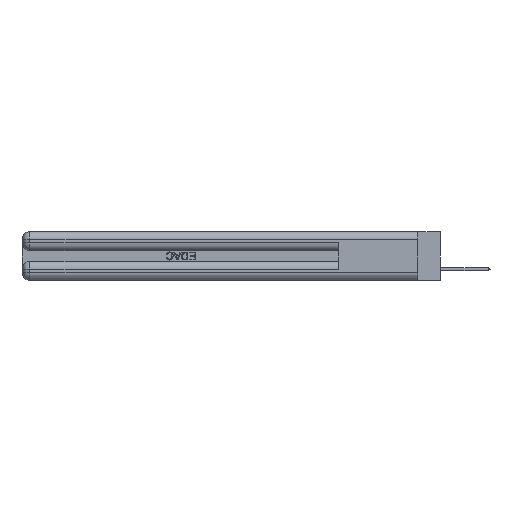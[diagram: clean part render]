
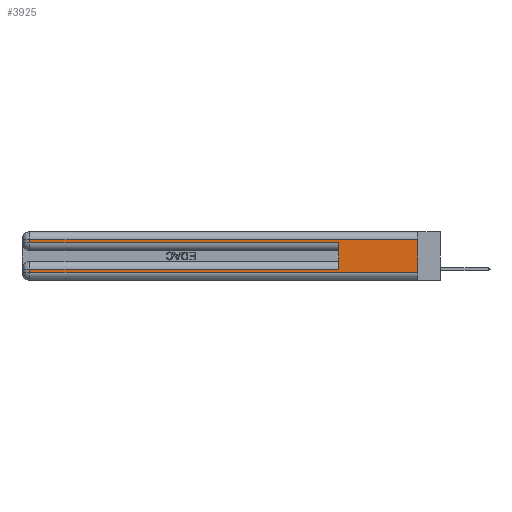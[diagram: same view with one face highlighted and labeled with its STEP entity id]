
A CAD part, left-side view. The second image highlights one B-rep face of the part: STEP entity #3925.
In plain terms, the highlighted planar face has unit normal (-1, 0, 0).
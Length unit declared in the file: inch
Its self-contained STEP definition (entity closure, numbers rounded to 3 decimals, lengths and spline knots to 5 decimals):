
#983 = ORIENTED_EDGE ( 'NONE', *, *, #35590, .T. ) ;
#3925 = ADVANCED_FACE ( 'NONE', ( #25614 ), #25757, .F. ) ;
#3992 = VERTEX_POINT ( 'NONE', #15371 ) ;
#4685 = DIRECTION ( 'NONE',  ( 0., 1., 0. ) ) ;
#4879 = CARTESIAN_POINT ( 'NONE',  ( 0., 2.94, 0.285 ) ) ;
#5951 = VERTEX_POINT ( 'NONE', #17149 ) ;
#6037 = VERTEX_POINT ( 'NONE', #38545 ) ;
#6633 = EDGE_CURVE ( 'NONE', #3992, #28101, #35765, .T. ) ;
#7548 = VERTEX_POINT ( 'NONE', #35885 ) ;
#9211 = LINE ( 'NONE', #29514, #38019 ) ;
#9677 = ORIENTED_EDGE ( 'NONE', *, *, #19985, .F. ) ;
#11271 = CARTESIAN_POINT ( 'NONE',  ( 0., 0., 0.37 ) ) ;
#12176 = EDGE_CURVE ( 'NONE', #13799, #7548, #9211, .T. ) ;
#12217 = DIRECTION ( 'NONE',  ( 0., 0., -1. ) ) ;
#12377 = DIRECTION ( 'NONE',  ( 0., 0., -1. ) ) ;
#12489 = LINE ( 'NONE', #27497, #17004 ) ;
#12563 = EDGE_CURVE ( 'NONE', #41067, #20176, #24419, .T. ) ;
#12713 = ORIENTED_EDGE ( 'NONE', *, *, #6633, .T. ) ;
#13020 = VECTOR ( 'NONE', #12377, 39.37008 ) ;
#13691 = CARTESIAN_POINT ( 'NONE',  ( 0., 0., 0.06 ) ) ;
#13745 = CARTESIAN_POINT ( 'NONE',  ( 0., 0.6, 0.285 ) ) ;
#13799 = VERTEX_POINT ( 'NONE', #23490 ) ;
#13914 = VECTOR ( 'NONE', #40086, 39.37008 ) ;
#14668 = EDGE_CURVE ( 'NONE', #7548, #3992, #42395, .T. ) ;
#14805 = VECTOR ( 'NONE', #18972, 39.37008 ) ;
#14844 = CARTESIAN_POINT ( 'NONE',  ( 0., 0.6, 0.145 ) ) ;
#15371 = CARTESIAN_POINT ( 'NONE',  ( 0., 2.94, 0.06 ) ) ;
#16921 = LINE ( 'NONE', #17027, #31066 ) ;
#17004 = VECTOR ( 'NONE', #45687, 39.37008 ) ;
#17027 = CARTESIAN_POINT ( 'NONE',  ( 0., 0., 0.31 ) ) ;
#17149 = CARTESIAN_POINT ( 'NONE',  ( 0., 0., 0.31 ) ) ;
#18445 = ORIENTED_EDGE ( 'NONE', *, *, #12176, .T. ) ;
#18704 = VECTOR ( 'NONE', #42557, 39.37008 ) ;
#18972 = DIRECTION ( 'NONE',  ( 0., -1., 0. ) ) ;
#19136 = CARTESIAN_POINT ( 'NONE',  ( 0., 0., 0.285 ) ) ;
#19985 = EDGE_CURVE ( 'NONE', #5951, #28101, #12489, .T. ) ;
#20176 = VERTEX_POINT ( 'NONE', #13745 ) ;
#22320 = LINE ( 'NONE', #14844, #13914 ) ;
#23490 = CARTESIAN_POINT ( 'NONE',  ( 0., 0.6, 0.085 ) ) ;
#23525 = EDGE_CURVE ( 'NONE', #13799, #20176, #22320, .T. ) ;
#24419 = LINE ( 'NONE', #19136, #14805 ) ;
#25614 = FACE_OUTER_BOUND ( 'NONE', #29400, .T. ) ;
#25757 = PLANE ( 'NONE',  #39024 ) ;
#25872 = ORIENTED_EDGE ( 'NONE', *, *, #12563, .T. ) ;
#26245 = LINE ( 'NONE', #45689, #26849 ) ;
#26849 = VECTOR ( 'NONE', #27986, 39.37008 ) ;
#27497 = CARTESIAN_POINT ( 'NONE',  ( 0., 0., 0.37 ) ) ;
#27986 = DIRECTION ( 'NONE',  ( 0., 0., -1. ) ) ;
#28101 = VERTEX_POINT ( 'NONE', #30935 ) ;
#29400 = EDGE_LOOP ( 'NONE', ( #9677, #983, #44951, #25872, #35628, #18445, #33652, #12713 ) ) ;
#29514 = CARTESIAN_POINT ( 'NONE',  ( 0., 0., 0.085 ) ) ;
#30935 = CARTESIAN_POINT ( 'NONE',  ( 0., 0., 0.06 ) ) ;
#31066 = VECTOR ( 'NONE', #42462, 39.37008 ) ;
#32209 = EDGE_CURVE ( 'NONE', #6037, #41067, #26245, .T. ) ;
#33652 = ORIENTED_EDGE ( 'NONE', *, *, #14668, .T. ) ;
#33838 = DIRECTION ( 'NONE',  ( 1., 0., 0. ) ) ;
#35590 = EDGE_CURVE ( 'NONE', #5951, #6037, #16921, .T. ) ;
#35628 = ORIENTED_EDGE ( 'NONE', *, *, #23525, .F. ) ;
#35765 = LINE ( 'NONE', #13691, #18704 ) ;
#35885 = CARTESIAN_POINT ( 'NONE',  ( 0., 2.94, 0.085 ) ) ;
#38019 = VECTOR ( 'NONE', #4685, 39.37008 ) ;
#38545 = CARTESIAN_POINT ( 'NONE',  ( 0., 2.94, 0.31 ) ) ;
#39024 = AXIS2_PLACEMENT_3D ( 'NONE', #11271, #33838, #12217 ) ;
#40086 = DIRECTION ( 'NONE',  ( 0., 0., 1. ) ) ;
#41067 = VERTEX_POINT ( 'NONE', #4879 ) ;
#42395 = LINE ( 'NONE', #43367, #13020 ) ;
#42462 = DIRECTION ( 'NONE',  ( 0., 1., 0. ) ) ;
#42557 = DIRECTION ( 'NONE',  ( 0., -1., 0. ) ) ;
#43367 = CARTESIAN_POINT ( 'NONE',  ( 0., 2.94, 0.37 ) ) ;
#44951 = ORIENTED_EDGE ( 'NONE', *, *, #32209, .T. ) ;
#45687 = DIRECTION ( 'NONE',  ( 0., 0., -1. ) ) ;
#45689 = CARTESIAN_POINT ( 'NONE',  ( 0., 2.94, 0.37 ) ) ;
